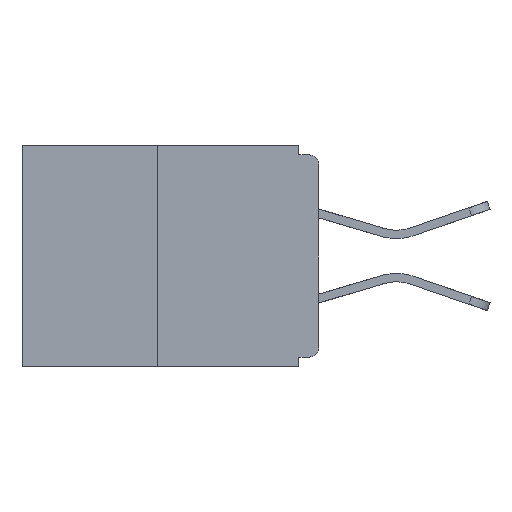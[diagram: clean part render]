
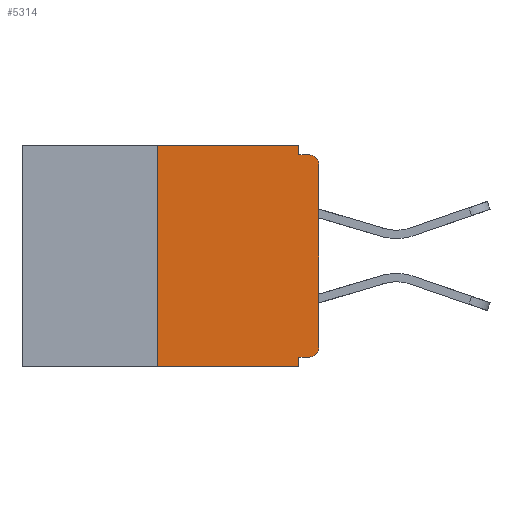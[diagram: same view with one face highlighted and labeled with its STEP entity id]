
A CAD part, left-side view. The second image highlights one B-rep face of the part: STEP entity #5314.
In plain terms, the highlighted planar face has unit normal (-1, 0, 0).
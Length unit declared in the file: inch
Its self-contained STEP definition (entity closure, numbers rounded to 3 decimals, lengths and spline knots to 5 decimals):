
#390 = VECTOR ( 'NONE', #612, 39.37008 ) ;
#612 = DIRECTION ( 'NONE',  ( 0., -1., 0. ) ) ;
#1010 = CARTESIAN_POINT ( 'NONE',  ( 0., 0.031, -0.015 ) ) ;
#1455 = EDGE_CURVE ( 'NONE', #10521, #18945, #6169, .T. ) ;
#1469 = CARTESIAN_POINT ( 'NONE',  ( 0., 0.015, -0.015 ) ) ;
#1483 = ORIENTED_EDGE ( 'NONE', *, *, #10481, .T. ) ;
#1656 = CARTESIAN_POINT ( 'NONE',  ( 0., 0.46, -0.343 ) ) ;
#1677 = CARTESIAN_POINT ( 'NONE',  ( 0., 0.46, 0. ) ) ;
#3708 = VECTOR ( 'NONE', #27139, 39.37008 ) ;
#4696 = CARTESIAN_POINT ( 'NONE',  ( 0., 0., -0.313 ) ) ;
#4729 = CARTESIAN_POINT ( 'NONE',  ( 0., 0., 0. ) ) ;
#5314 = ADVANCED_FACE ( 'NONE', ( #12256 ), #16608, .F. ) ;
#5432 = VECTOR ( 'NONE', #6932, 39.37008 ) ;
#6169 = LINE ( 'NONE', #15797, #390 ) ;
#6665 = CARTESIAN_POINT ( 'NONE',  ( 0., 0.25, -0.343 ) ) ;
#6932 = DIRECTION ( 'NONE',  ( 0., 0., 1. ) ) ;
#6981 = EDGE_CURVE ( 'NONE', #9362, #21145, #11170, .T. ) ;
#7154 = DIRECTION ( 'NONE',  ( -1., 0., 0. ) ) ;
#7741 = CARTESIAN_POINT ( 'NONE',  ( 0., 0., -0.015 ) ) ;
#8374 = VERTEX_POINT ( 'NONE', #1469 ) ;
#8692 = VERTEX_POINT ( 'NONE', #17190 ) ;
#8808 = CARTESIAN_POINT ( 'NONE',  ( 0., 0.031, 0. ) ) ;
#9222 = DIRECTION ( 'NONE',  ( 0., 0., -1. ) ) ;
#9326 = DIRECTION ( 'NONE',  ( 0., 0., -1. ) ) ;
#9362 = VERTEX_POINT ( 'NONE', #4696 ) ;
#9375 = DIRECTION ( 'NONE',  ( -1., 0., 0. ) ) ;
#9981 = EDGE_CURVE ( 'NONE', #18945, #23024, #26149, .T. ) ;
#10368 = LINE ( 'NONE', #22086, #20856 ) ;
#10481 = EDGE_CURVE ( 'NONE', #24045, #17384, #19674, .T. ) ;
#10521 = VERTEX_POINT ( 'NONE', #19476 ) ;
#10837 = ORIENTED_EDGE ( 'NONE', *, *, #14315, .F. ) ;
#10918 = EDGE_CURVE ( 'NONE', #23024, #8374, #16945, .T. ) ;
#11170 = LINE ( 'NONE', #4729, #5432 ) ;
#11288 = CARTESIAN_POINT ( 'NONE',  ( 0., 0.031, -0.343 ) ) ;
#11291 = CARTESIAN_POINT ( 'NONE',  ( 0., 0.031, 0. ) ) ;
#11377 = CIRCLE ( 'NONE', #23832, 0.015 ) ;
#11387 = CARTESIAN_POINT ( 'NONE',  ( 0., 0.015, -0.03 ) ) ;
#12256 = FACE_OUTER_BOUND ( 'NONE', #22857, .T. ) ;
#12697 = ORIENTED_EDGE ( 'NONE', *, *, #25537, .F. ) ;
#12843 = AXIS2_PLACEMENT_3D ( 'NONE', #1677, #25552, #25462 ) ;
#12884 = VECTOR ( 'NONE', #21080, 39.37008 ) ;
#13066 = EDGE_CURVE ( 'NONE', #24045, #10521, #10368, .T. ) ;
#13075 = EDGE_CURVE ( 'NONE', #21145, #8374, #11377, .T. ) ;
#13359 = LINE ( 'NONE', #14808, #15380 ) ;
#13401 = VERTEX_POINT ( 'NONE', #25663 ) ;
#14104 = CIRCLE ( 'NONE', #17909, 0.015 ) ;
#14130 = VECTOR ( 'NONE', #9222, 39.37008 ) ;
#14315 = EDGE_CURVE ( 'NONE', #8692, #13401, #13359, .T. ) ;
#14808 = CARTESIAN_POINT ( 'NONE',  ( 0., 0., -0.328 ) ) ;
#14890 = ORIENTED_EDGE ( 'NONE', *, *, #9981, .F. ) ;
#14965 = VECTOR ( 'NONE', #19775, 39.37008 ) ;
#15380 = VECTOR ( 'NONE', #25054, 39.37008 ) ;
#15386 = ORIENTED_EDGE ( 'NONE', *, *, #13075, .T. ) ;
#15797 = CARTESIAN_POINT ( 'NONE',  ( 0., 0.46, 0. ) ) ;
#16608 = PLANE ( 'NONE',  #12843 ) ;
#16945 = LINE ( 'NONE', #7741, #3708 ) ;
#17190 = CARTESIAN_POINT ( 'NONE',  ( 0., 0.015, -0.328 ) ) ;
#17384 = VERTEX_POINT ( 'NONE', #26299 ) ;
#17909 = AXIS2_PLACEMENT_3D ( 'NONE', #22328, #9375, #24509 ) ;
#18945 = VERTEX_POINT ( 'NONE', #11291 ) ;
#19194 = LINE ( 'NONE', #11288, #14130 ) ;
#19476 = CARTESIAN_POINT ( 'NONE',  ( 0., 0.25, 0. ) ) ;
#19674 = LINE ( 'NONE', #1656, #12884 ) ;
#19775 = DIRECTION ( 'NONE',  ( 0., 0., -1. ) ) ;
#20856 = VECTOR ( 'NONE', #24270, 39.37008 ) ;
#20997 = ORIENTED_EDGE ( 'NONE', *, *, #25787, .T. ) ;
#21080 = DIRECTION ( 'NONE',  ( 0., -1., 0. ) ) ;
#21145 = VERTEX_POINT ( 'NONE', #25622 ) ;
#22086 = CARTESIAN_POINT ( 'NONE',  ( 0., 0.25, 0. ) ) ;
#22328 = CARTESIAN_POINT ( 'NONE',  ( 0., 0.015, -0.313 ) ) ;
#22360 = ORIENTED_EDGE ( 'NONE', *, *, #13066, .F. ) ;
#22857 = EDGE_LOOP ( 'NONE', ( #25924, #22360, #1483, #12697, #10837, #20997, #24119, #15386, #23647, #14890 ) ) ;
#23024 = VERTEX_POINT ( 'NONE', #1010 ) ;
#23647 = ORIENTED_EDGE ( 'NONE', *, *, #10918, .F. ) ;
#23832 = AXIS2_PLACEMENT_3D ( 'NONE', #11387, #7154, #9326 ) ;
#24045 = VERTEX_POINT ( 'NONE', #6665 ) ;
#24119 = ORIENTED_EDGE ( 'NONE', *, *, #6981, .T. ) ;
#24270 = DIRECTION ( 'NONE',  ( 0., 0., 1. ) ) ;
#24509 = DIRECTION ( 'NONE',  ( 0., 0., -1. ) ) ;
#25054 = DIRECTION ( 'NONE',  ( 0., 1., 0. ) ) ;
#25462 = DIRECTION ( 'NONE',  ( 0., 0., -1. ) ) ;
#25537 = EDGE_CURVE ( 'NONE', #13401, #17384, #19194, .T. ) ;
#25552 = DIRECTION ( 'NONE',  ( 1., 0., 0. ) ) ;
#25622 = CARTESIAN_POINT ( 'NONE',  ( 0., 0., -0.03 ) ) ;
#25663 = CARTESIAN_POINT ( 'NONE',  ( 0., 0.031, -0.328 ) ) ;
#25787 = EDGE_CURVE ( 'NONE', #8692, #9362, #14104, .T. ) ;
#25924 = ORIENTED_EDGE ( 'NONE', *, *, #1455, .F. ) ;
#26149 = LINE ( 'NONE', #8808, #14965 ) ;
#26299 = CARTESIAN_POINT ( 'NONE',  ( 0., 0.031, -0.343 ) ) ;
#27139 = DIRECTION ( 'NONE',  ( 0., -1., 0. ) ) ;
